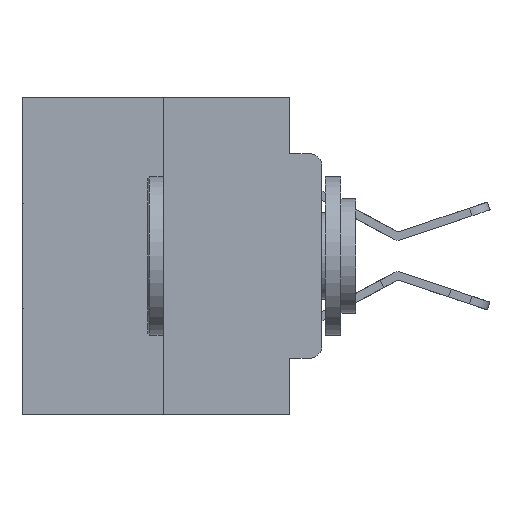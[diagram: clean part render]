
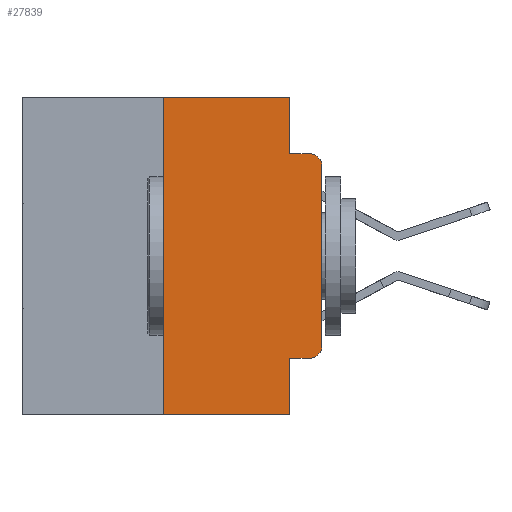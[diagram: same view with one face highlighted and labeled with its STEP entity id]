
A CAD part, left-side view. The second image highlights one B-rep face of the part: STEP entity #27839.
In plain terms, the highlighted planar face has unit normal (-1, 0, 0).
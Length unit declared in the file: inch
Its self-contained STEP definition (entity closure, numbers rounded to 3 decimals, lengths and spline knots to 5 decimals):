
#472 = VERTEX_POINT ( 'NONE', #8743 ) ;
#753 = AXIS2_PLACEMENT_3D ( 'NONE', #13163, #28358, #15431 ) ;
#766 = DIRECTION ( 'NONE',  ( 0., -1., 0. ) ) ;
#846 = VERTEX_POINT ( 'NONE', #10402 ) ;
#939 = VERTEX_POINT ( 'NONE', #8774 ) ;
#1683 = DIRECTION ( 'NONE',  ( 0., 0., 1. ) ) ;
#1720 = ORIENTED_EDGE ( 'NONE', *, *, #26363, .F. ) ;
#2556 = EDGE_CURVE ( 'NONE', #17202, #846, #17255, .T. ) ;
#2700 = CARTESIAN_POINT ( 'NONE',  ( 0., 0.25, -0.5 ) ) ;
#3777 = VERTEX_POINT ( 'NONE', #27882 ) ;
#4712 = FACE_OUTER_BOUND ( 'NONE', #9683, .T. ) ;
#5084 = VECTOR ( 'NONE', #24680, 39.37008 ) ;
#5441 = CARTESIAN_POINT ( 'NONE',  ( 0., 0.473, 0. ) ) ;
#5883 = CARTESIAN_POINT ( 'NONE',  ( 0., 0., -0.3915 ) ) ;
#6014 = VECTOR ( 'NONE', #766, 39.37008 ) ;
#6117 = CARTESIAN_POINT ( 'NONE',  ( 0., 0.25, 0. ) ) ;
#6291 = ORIENTED_EDGE ( 'NONE', *, *, #8223, .T. ) ;
#6802 = AXIS2_PLACEMENT_3D ( 'NONE', #5441, #20925, #7642 ) ;
#6946 = VECTOR ( 'NONE', #12182, 39.37008 ) ;
#7642 = DIRECTION ( 'NONE',  ( 0., 0., -1. ) ) ;
#8223 = EDGE_CURVE ( 'NONE', #846, #939, #22394, .T. ) ;
#8602 = CIRCLE ( 'NONE', #19996, 0.02 ) ;
#8743 = CARTESIAN_POINT ( 'NONE',  ( 0., 0.02, -0.4115 ) ) ;
#8774 = CARTESIAN_POINT ( 'NONE',  ( 0., 0.02, -0.0885 ) ) ;
#8888 = CARTESIAN_POINT ( 'NONE',  ( 0., 0.051, -0.4115 ) ) ;
#8967 = EDGE_CURVE ( 'NONE', #13871, #10243, #16928, .T. ) ;
#9330 = CARTESIAN_POINT ( 'NONE',  ( 0., 0.051, 0. ) ) ;
#9563 = VECTOR ( 'NONE', #1683, 39.37008 ) ;
#9655 = LINE ( 'NONE', #23316, #26431 ) ;
#9683 = EDGE_LOOP ( 'NONE', ( #17457, #6291, #18142, #18811, #1720, #25245, #20212, #15082, #21563, #11229 ) ) ;
#10243 = VERTEX_POINT ( 'NONE', #24802 ) ;
#10402 = CARTESIAN_POINT ( 'NONE',  ( 0., 0., -0.1085 ) ) ;
#11105 = LINE ( 'NONE', #11321, #25794 ) ;
#11229 = ORIENTED_EDGE ( 'NONE', *, *, #26624, .T. ) ;
#11321 = CARTESIAN_POINT ( 'NONE',  ( 0., 0.051, -0.0885 ) ) ;
#12182 = DIRECTION ( 'NONE',  ( 0., 0., -1. ) ) ;
#12308 = LINE ( 'NONE', #17854, #23301 ) ;
#12600 = EDGE_CURVE ( 'NONE', #21616, #26819, #18790, .T. ) ;
#12795 = CARTESIAN_POINT ( 'NONE',  ( 0., 0.02, -0.3915 ) ) ;
#13163 = CARTESIAN_POINT ( 'NONE',  ( 0., 0.02, -0.1085 ) ) ;
#13374 = DIRECTION ( 'NONE',  ( 0., 0., 1. ) ) ;
#13529 = CARTESIAN_POINT ( 'NONE',  ( 0., 0., 0. ) ) ;
#13871 = VERTEX_POINT ( 'NONE', #16622 ) ;
#14251 = VERTEX_POINT ( 'NONE', #2700 ) ;
#14467 = DIRECTION ( 'NONE',  ( 0., -1., 0. ) ) ;
#14813 = EDGE_CURVE ( 'NONE', #10243, #939, #11105, .T. ) ;
#15072 = DIRECTION ( 'NONE',  ( 0., 0., -1. ) ) ;
#15082 = ORIENTED_EDGE ( 'NONE', *, *, #12600, .F. ) ;
#15431 = DIRECTION ( 'NONE',  ( 0., 0., -1. ) ) ;
#16622 = CARTESIAN_POINT ( 'NONE',  ( 0., 0.051, 0. ) ) ;
#16628 = EDGE_CURVE ( 'NONE', #14251, #3777, #26996, .T. ) ;
#16928 = LINE ( 'NONE', #9330, #5084 ) ;
#17202 = VERTEX_POINT ( 'NONE', #5883 ) ;
#17255 = LINE ( 'NONE', #13529, #28032 ) ;
#17457 = ORIENTED_EDGE ( 'NONE', *, *, #2556, .T. ) ;
#17854 = CARTESIAN_POINT ( 'NONE',  ( 0., 0.473, -0.5 ) ) ;
#18013 = DIRECTION ( 'NONE',  ( 0., -1., 0. ) ) ;
#18142 = ORIENTED_EDGE ( 'NONE', *, *, #14813, .F. ) ;
#18790 = LINE ( 'NONE', #18977, #6946 ) ;
#18811 = ORIENTED_EDGE ( 'NONE', *, *, #8967, .F. ) ;
#18977 = CARTESIAN_POINT ( 'NONE',  ( 0., 0.051, 0. ) ) ;
#19996 = AXIS2_PLACEMENT_3D ( 'NONE', #12795, #28012, #15072 ) ;
#20041 = DIRECTION ( 'NONE',  ( 0., -1., 0. ) ) ;
#20212 = ORIENTED_EDGE ( 'NONE', *, *, #26012, .T. ) ;
#20552 = EDGE_CURVE ( 'NONE', #21616, #472, #24289, .T. ) ;
#20925 = DIRECTION ( 'NONE',  ( 1., 0., 0. ) ) ;
#21563 = ORIENTED_EDGE ( 'NONE', *, *, #20552, .T. ) ;
#21616 = VERTEX_POINT ( 'NONE', #8888 ) ;
#22394 = CIRCLE ( 'NONE', #753, 0.02 ) ;
#22898 = CARTESIAN_POINT ( 'NONE',  ( 0., 0.051, -0.4115 ) ) ;
#23301 = VECTOR ( 'NONE', #20041, 39.37008 ) ;
#23316 = CARTESIAN_POINT ( 'NONE',  ( 0., 0.473, 0. ) ) ;
#24289 = LINE ( 'NONE', #22898, #6014 ) ;
#24359 = CARTESIAN_POINT ( 'NONE',  ( 0., 0.051, -0.5 ) ) ;
#24680 = DIRECTION ( 'NONE',  ( 0., 0., -1. ) ) ;
#24802 = CARTESIAN_POINT ( 'NONE',  ( 0., 0.051, -0.0885 ) ) ;
#25245 = ORIENTED_EDGE ( 'NONE', *, *, #16628, .F. ) ;
#25794 = VECTOR ( 'NONE', #18013, 39.37008 ) ;
#26012 = EDGE_CURVE ( 'NONE', #14251, #26819, #12308, .T. ) ;
#26090 = PLANE ( 'NONE',  #6802 ) ;
#26363 = EDGE_CURVE ( 'NONE', #3777, #13871, #9655, .T. ) ;
#26431 = VECTOR ( 'NONE', #14467, 39.37008 ) ;
#26624 = EDGE_CURVE ( 'NONE', #472, #17202, #8602, .T. ) ;
#26819 = VERTEX_POINT ( 'NONE', #24359 ) ;
#26996 = LINE ( 'NONE', #6117, #9563 ) ;
#27839 = ADVANCED_FACE ( 'NONE', ( #4712 ), #26090, .F. ) ;
#27882 = CARTESIAN_POINT ( 'NONE',  ( 0., 0.25, 0. ) ) ;
#28012 = DIRECTION ( 'NONE',  ( -1., 0., 0. ) ) ;
#28032 = VECTOR ( 'NONE', #13374, 39.37008 ) ;
#28358 = DIRECTION ( 'NONE',  ( -1., 0., 0. ) ) ;
